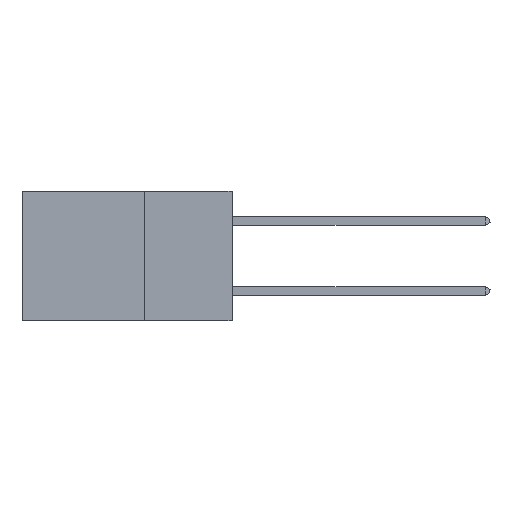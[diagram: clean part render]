
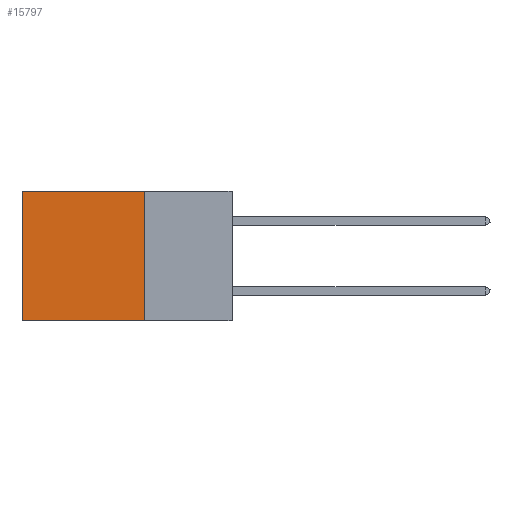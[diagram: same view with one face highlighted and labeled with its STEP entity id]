
A CAD part, left-side view. The second image highlights one B-rep face of the part: STEP entity #15797.
In plain terms, the highlighted planar face has unit normal (-1, 0, 0).
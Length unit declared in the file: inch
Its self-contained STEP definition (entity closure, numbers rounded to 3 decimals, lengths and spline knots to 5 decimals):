
#293 = VECTOR ( 'NONE', #22240, 39.37008 ) ;
#821 = ORIENTED_EDGE ( 'NONE', *, *, #24324, .T. ) ;
#1122 = DIRECTION ( 'NONE',  ( 0., 0., -1. ) ) ;
#2203 = DIRECTION ( 'NONE',  ( 1., 0., 0. ) ) ;
#3257 = CARTESIAN_POINT ( 'NONE',  ( 0.2875, 0.25, -0.37 ) ) ;
#4917 = LINE ( 'NONE', #24983, #16804 ) ;
#5041 = ORIENTED_EDGE ( 'NONE', *, *, #13940, .F. ) ;
#5952 = ORIENTED_EDGE ( 'NONE', *, *, #15483, .T. ) ;
#6920 = CARTESIAN_POINT ( 'NONE',  ( 0.2875, 0.25, -0.37 ) ) ;
#7579 = EDGE_LOOP ( 'NONE', ( #821, #16396, #5041, #5952 ) ) ;
#8713 = VERTEX_POINT ( 'NONE', #14966 ) ;
#9066 = VERTEX_POINT ( 'NONE', #24933 ) ;
#9843 = VECTOR ( 'NONE', #1122, 39.37008 ) ;
#9871 = DIRECTION ( 'NONE',  ( 0., 0., -1. ) ) ;
#10105 = FACE_OUTER_BOUND ( 'NONE', #7579, .T. ) ;
#12482 = CARTESIAN_POINT ( 'NONE',  ( 0.2875, 0.25, 0. ) ) ;
#13940 = EDGE_CURVE ( 'NONE', #8713, #26115, #4917, .T. ) ;
#14720 = AXIS2_PLACEMENT_3D ( 'NONE', #19872, #2203, #17824 ) ;
#14966 = CARTESIAN_POINT ( 'NONE',  ( 0.2875, 0.25, 0. ) ) ;
#15483 = EDGE_CURVE ( 'NONE', #8713, #9066, #17695, .T. ) ;
#15665 = PLANE ( 'NONE',  #14720 ) ;
#15797 = ADVANCED_FACE ( 'NONE', ( #10105 ), #15665, .F. ) ;
#16396 = ORIENTED_EDGE ( 'NONE', *, *, #21209, .F. ) ;
#16450 = LINE ( 'NONE', #23148, #9843 ) ;
#16804 = VECTOR ( 'NONE', #9871, 39.37008 ) ;
#16917 = DIRECTION ( 'NONE',  ( 0., 1., 0. ) ) ;
#17695 = LINE ( 'NONE', #12482, #28118 ) ;
#17824 = DIRECTION ( 'NONE',  ( 0., 0., -1. ) ) ;
#19872 = CARTESIAN_POINT ( 'NONE',  ( 0.2875, 0.25, 0. ) ) ;
#19883 = VERTEX_POINT ( 'NONE', #23725 ) ;
#21209 = EDGE_CURVE ( 'NONE', #26115, #19883, #27941, .T. ) ;
#22240 = DIRECTION ( 'NONE',  ( 0., 1., 0. ) ) ;
#23148 = CARTESIAN_POINT ( 'NONE',  ( 0.2875, 0.6, 0. ) ) ;
#23725 = CARTESIAN_POINT ( 'NONE',  ( 0.2875, 0.6, -0.37 ) ) ;
#24324 = EDGE_CURVE ( 'NONE', #9066, #19883, #16450, .T. ) ;
#24933 = CARTESIAN_POINT ( 'NONE',  ( 0.2875, 0.6, 0. ) ) ;
#24983 = CARTESIAN_POINT ( 'NONE',  ( 0.2875, 0.25, 0. ) ) ;
#26115 = VERTEX_POINT ( 'NONE', #3257 ) ;
#27941 = LINE ( 'NONE', #6920, #293 ) ;
#28118 = VECTOR ( 'NONE', #16917, 39.37008 ) ;
